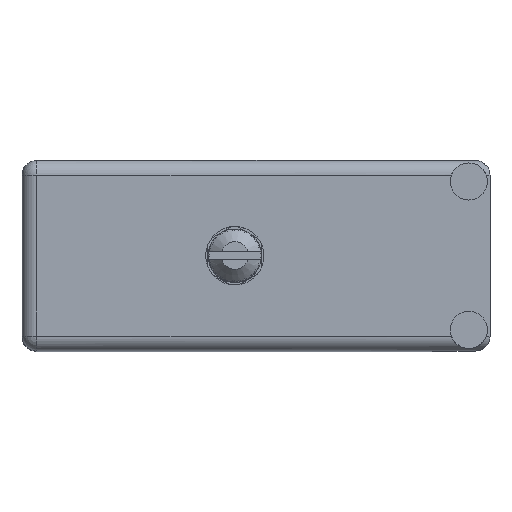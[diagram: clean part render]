
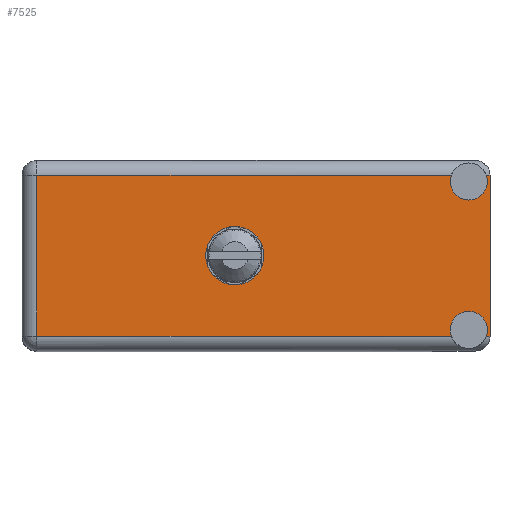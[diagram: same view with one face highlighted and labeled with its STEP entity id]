
A CAD part, top view. The second image highlights one B-rep face of the part: STEP entity #7525.
In plain terms, the highlighted face is planar.
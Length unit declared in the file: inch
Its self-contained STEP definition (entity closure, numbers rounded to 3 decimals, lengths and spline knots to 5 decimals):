
#525 = EDGE_CURVE ( 'NONE', #40263, #50560, #52736, .T. ) ;
#3579 = AXIS2_PLACEMENT_3D ( 'NONE', #16902, #41178, #88826 ) ;
#3876 = EDGE_CURVE ( 'NONE', #91215, #67013, #62685, .T. ) ;
#4277 = FACE_BOUND ( 'NONE', #5715, .T. ) ;
#5344 = VECTOR ( 'NONE', #35532, 39.37008 ) ;
#5715 = EDGE_LOOP ( 'NONE', ( #56669, #39099 ) ) ;
#6662 = CARTESIAN_POINT ( 'NONE',  ( 1.004, 1.566, -0.587 ) ) ;
#7525 = ADVANCED_FACE ( 'NONE', ( #4277, #68574 ), #56383, .T. ) ;
#8081 = DIRECTION ( 'NONE',  ( 0., 1., 0. ) ) ;
#8664 = AXIS2_PLACEMENT_3D ( 'NONE', #60262, #51752, #11951 ) ;
#9080 = CARTESIAN_POINT ( 'NONE',  ( 2.208, 1.566, -0.829 ) ) ;
#9121 = VECTOR ( 'NONE', #72707, 39.37008 ) ;
#9367 = CARTESIAN_POINT ( 'NONE',  ( 2.208, 1.566, -0.07 ) ) ;
#9839 = CARTESIAN_POINT ( 'NONE',  ( 0.07, 1.566, -0.899 ) ) ;
#11951 = DIRECTION ( 'NONE',  ( 0., 0., 1. ) ) ;
#11975 = CIRCLE ( 'NONE', #13239, 0.0875 ) ;
#12731 = CIRCLE ( 'NONE', #25601, 0.0875 ) ;
#13239 = AXIS2_PLACEMENT_3D ( 'NONE', #36271, #101815, #45098 ) ;
#14127 = DIRECTION ( 'NONE',  ( 0., 0., 1. ) ) ;
#14652 = AXIS2_PLACEMENT_3D ( 'NONE', #64473, #8081, #81038 ) ;
#15876 = EDGE_CURVE ( 'NONE', #55292, #72029, #24219, .T. ) ;
#16834 = LINE ( 'NONE', #95350, #9121 ) ;
#16902 = CARTESIAN_POINT ( 'NONE',  ( 2.108, 1.566, -0.0995 ) ) ;
#17592 = EDGE_CURVE ( 'NONE', #50560, #97661, #12731, .T. ) ;
#19322 = CARTESIAN_POINT ( 'NONE',  ( 2.208, 1.566, 0. ) ) ;
#21515 = VECTOR ( 'NONE', #57088, 39.37008 ) ;
#23442 = VERTEX_POINT ( 'NONE', #32363 ) ;
#24034 = LINE ( 'NONE', #9839, #21515 ) ;
#24219 = LINE ( 'NONE', #19322, #5344 ) ;
#24682 = ORIENTED_EDGE ( 'NONE', *, *, #3876, .F. ) ;
#25601 = AXIS2_PLACEMENT_3D ( 'NONE', #36505, #77055, #46017 ) ;
#28837 = CARTESIAN_POINT ( 'NONE',  ( 2.19038, 1.566, -0.07 ) ) ;
#29399 = CARTESIAN_POINT ( 'NONE',  ( 2.208, 1.566, -0.07 ) ) ;
#29538 = VERTEX_POINT ( 'NONE', #74431 ) ;
#29931 = AXIS2_PLACEMENT_3D ( 'NONE', #38417, #62807, #71913 ) ;
#30013 = CARTESIAN_POINT ( 'NONE',  ( 0.07, 1.566, -0.829 ) ) ;
#32363 = CARTESIAN_POINT ( 'NONE',  ( 0.07, 1.566, -0.07 ) ) ;
#34272 = CARTESIAN_POINT ( 'NONE',  ( 2.108, 1.566, -0.187 ) ) ;
#35532 = DIRECTION ( 'NONE',  ( 0., 0., 1. ) ) ;
#36271 = CARTESIAN_POINT ( 'NONE',  ( 2.108, 1.566, -0.0995 ) ) ;
#36505 = CARTESIAN_POINT ( 'NONE',  ( 2.108, 1.566, -0.7995 ) ) ;
#38417 = CARTESIAN_POINT ( 'NONE',  ( 1.004, 1.566, -0.4495 ) ) ;
#39081 = VERTEX_POINT ( 'NONE', #28837 ) ;
#39099 = ORIENTED_EDGE ( 'NONE', *, *, #48240, .F. ) ;
#40263 = VERTEX_POINT ( 'NONE', #54446 ) ;
#41178 = DIRECTION ( 'NONE',  ( 0., 1., 0. ) ) ;
#41438 = EDGE_CURVE ( 'NONE', #55292, #97661, #16834, .T. ) ;
#45098 = DIRECTION ( 'NONE',  ( 0., 0., 1. ) ) ;
#46017 = DIRECTION ( 'NONE',  ( 0., 0., 1. ) ) ;
#48240 = EDGE_CURVE ( 'NONE', #90349, #29538, #93794, .T. ) ;
#48488 = DIRECTION ( 'NONE',  ( -1., 0., 0. ) ) ;
#49547 = DIRECTION ( 'NONE',  ( 1., 0., 0. ) ) ;
#50249 = VECTOR ( 'NONE', #48488, 39.37008 ) ;
#50560 = VERTEX_POINT ( 'NONE', #95441 ) ;
#51752 = DIRECTION ( 'NONE',  ( 0., 1., 0. ) ) ;
#52736 = CIRCLE ( 'NONE', #8664, 0.0875 ) ;
#54446 = CARTESIAN_POINT ( 'NONE',  ( 2.02562, 1.566, -0.829 ) ) ;
#55055 = ORIENTED_EDGE ( 'NONE', *, *, #41438, .T. ) ;
#55241 = ORIENTED_EDGE ( 'NONE', *, *, #82003, .T. ) ;
#55292 = VERTEX_POINT ( 'NONE', #9080 ) ;
#56383 = PLANE ( 'NONE',  #14652 ) ;
#56669 = ORIENTED_EDGE ( 'NONE', *, *, #63577, .F. ) ;
#57088 = DIRECTION ( 'NONE',  ( 0., 0., 1. ) ) ;
#60262 = CARTESIAN_POINT ( 'NONE',  ( 2.108, 1.566, -0.7995 ) ) ;
#60544 = EDGE_LOOP ( 'NONE', ( #55241, #24682, #60905, #86181, #80211, #55055, #62400, #74536, #84183, #76704 ) ) ;
#60905 = ORIENTED_EDGE ( 'NONE', *, *, #71001, .F. ) ;
#61625 = LINE ( 'NONE', #65417, #50249 ) ;
#62400 = ORIENTED_EDGE ( 'NONE', *, *, #17592, .F. ) ;
#62685 = CIRCLE ( 'NONE', #3579, 0.0875 ) ;
#62766 = DIRECTION ( 'NONE',  ( 0., 1., 0. ) ) ;
#62807 = DIRECTION ( 'NONE',  ( 0., 1., 0. ) ) ;
#63577 = EDGE_CURVE ( 'NONE', #29538, #90349, #101024, .T. ) ;
#64473 = CARTESIAN_POINT ( 'NONE',  ( 0., 1.566, -0.899 ) ) ;
#64544 = CARTESIAN_POINT ( 'NONE',  ( 2.02562, 1.566, -0.07 ) ) ;
#65417 = CARTESIAN_POINT ( 'NONE',  ( 0., 1.566, -0.829 ) ) ;
#66860 = VECTOR ( 'NONE', #49547, 39.37008 ) ;
#67013 = VERTEX_POINT ( 'NONE', #64544 ) ;
#68574 = FACE_OUTER_BOUND ( 'NONE', #60544, .T. ) ;
#71001 = EDGE_CURVE ( 'NONE', #39081, #91215, #11975, .T. ) ;
#71913 = DIRECTION ( 'NONE',  ( 0., 0., 1. ) ) ;
#72029 = VERTEX_POINT ( 'NONE', #29399 ) ;
#72707 = DIRECTION ( 'NONE',  ( -1., 0., 0. ) ) ;
#74431 = CARTESIAN_POINT ( 'NONE',  ( 1.004, 1.566, -0.312 ) ) ;
#74473 = AXIS2_PLACEMENT_3D ( 'NONE', #78609, #62766, #14127 ) ;
#74536 = ORIENTED_EDGE ( 'NONE', *, *, #525, .F. ) ;
#76704 = ORIENTED_EDGE ( 'NONE', *, *, #92839, .T. ) ;
#77055 = DIRECTION ( 'NONE',  ( 0., 1., 0. ) ) ;
#77746 = CARTESIAN_POINT ( 'NONE',  ( 2.208, 1.566, -0.07 ) ) ;
#78609 = CARTESIAN_POINT ( 'NONE',  ( 1.004, 1.566, -0.4495 ) ) ;
#79223 = LINE ( 'NONE', #77746, #100686 ) ;
#80211 = ORIENTED_EDGE ( 'NONE', *, *, #15876, .F. ) ;
#81038 = DIRECTION ( 'NONE',  ( 0., 0., 1. ) ) ;
#82003 = EDGE_CURVE ( 'NONE', #23442, #67013, #79223, .T. ) ;
#83941 = VERTEX_POINT ( 'NONE', #30013 ) ;
#84183 = ORIENTED_EDGE ( 'NONE', *, *, #94797, .T. ) ;
#85769 = LINE ( 'NONE', #9367, #66860 ) ;
#86181 = ORIENTED_EDGE ( 'NONE', *, *, #87578, .T. ) ;
#87578 = EDGE_CURVE ( 'NONE', #39081, #72029, #85769, .T. ) ;
#88338 = CARTESIAN_POINT ( 'NONE',  ( 2.19038, 1.566, -0.829 ) ) ;
#88826 = DIRECTION ( 'NONE',  ( 0., 0., 1. ) ) ;
#90349 = VERTEX_POINT ( 'NONE', #6662 ) ;
#91215 = VERTEX_POINT ( 'NONE', #34272 ) ;
#92839 = EDGE_CURVE ( 'NONE', #83941, #23442, #24034, .T. ) ;
#93794 = CIRCLE ( 'NONE', #29931, 0.1375 ) ;
#94797 = EDGE_CURVE ( 'NONE', #40263, #83941, #61625, .T. ) ;
#95350 = CARTESIAN_POINT ( 'NONE',  ( 0., 1.566, -0.829 ) ) ;
#95441 = CARTESIAN_POINT ( 'NONE',  ( 2.108, 1.566, -0.712 ) ) ;
#97661 = VERTEX_POINT ( 'NONE', #88338 ) ;
#100686 = VECTOR ( 'NONE', #102754, 39.37008 ) ;
#101024 = CIRCLE ( 'NONE', #74473, 0.1375 ) ;
#101815 = DIRECTION ( 'NONE',  ( 0., 1., 0. ) ) ;
#102754 = DIRECTION ( 'NONE',  ( 1., 0., 0. ) ) ;
